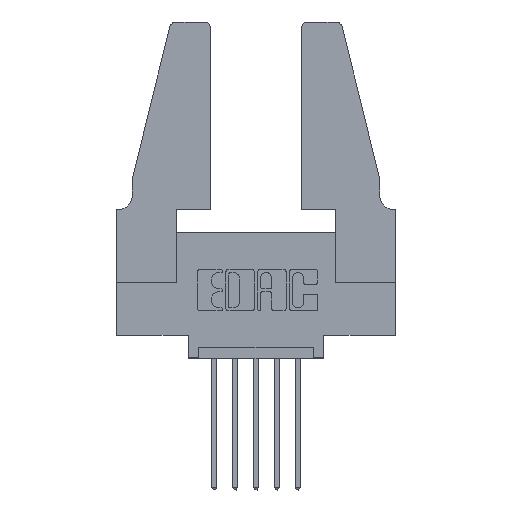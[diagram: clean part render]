
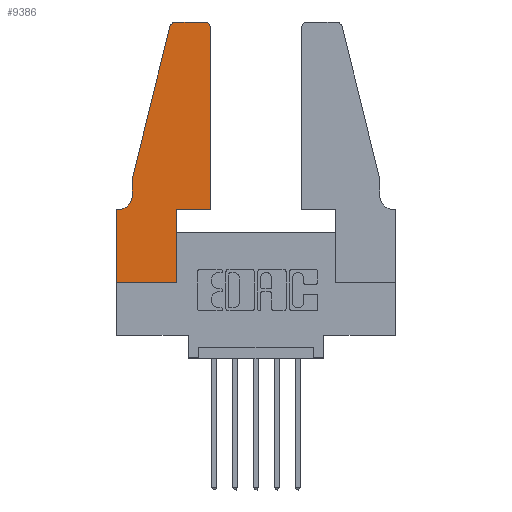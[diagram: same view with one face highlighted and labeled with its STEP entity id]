
A CAD part, top view. The second image highlights one B-rep face of the part: STEP entity #9386.
In plain terms, the highlighted planar face has unit normal (0, 0, 1).
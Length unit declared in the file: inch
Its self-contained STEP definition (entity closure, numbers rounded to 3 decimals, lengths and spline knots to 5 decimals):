
#49 = FACE_OUTER_BOUND ( 'NONE', #9135, .T. ) ;
#96 = EDGE_CURVE ( 'NONE', #5840, #1678, #9204, .T. ) ;
#103 = AXIS2_PLACEMENT_3D ( 'NONE', #2315, #10703, #559 ) ;
#222 = CARTESIAN_POINT ( 'NONE',  ( 0., 0.35, 0.37 ) ) ;
#270 = CARTESIAN_POINT ( 'NONE',  ( 0.4505, 0.35, 0.37 ) ) ;
#273 = VERTEX_POINT ( 'NONE', #8104 ) ;
#385 = AXIS2_PLACEMENT_3D ( 'NONE', #4995, #5031, #11006 ) ;
#559 = DIRECTION ( 'NONE',  ( 1., 0., 0. ) ) ;
#604 = DIRECTION ( 'NONE',  ( 0., -1., 0. ) ) ;
#610 = AXIS2_PLACEMENT_3D ( 'NONE', #1823, #6894, #1903 ) ;
#1371 = CARTESIAN_POINT ( 'NONE',  ( 0.0755, 0.5, 0.37 ) ) ;
#1377 = LINE ( 'NONE', #1539, #10598 ) ;
#1414 = EDGE_CURVE ( 'NONE', #4441, #5283, #2068, .T. ) ;
#1539 = CARTESIAN_POINT ( 'NONE',  ( 0.4505, 0.35, 0.37 ) ) ;
#1623 = VERTEX_POINT ( 'NONE', #5272 ) ;
#1678 = VERTEX_POINT ( 'NONE', #5343 ) ;
#1774 = CARTESIAN_POINT ( 'NONE',  ( 0.25487, 1.22718, 0.37 ) ) ;
#1823 = CARTESIAN_POINT ( 'NONE',  ( 0.284, 1.22, 0.37 ) ) ;
#1831 = VECTOR ( 'NONE', #3456, 39.37008 ) ;
#1847 = PLANE ( 'NONE',  #2096 ) ;
#1903 = DIRECTION ( 'NONE',  ( 1., 0., 0. ) ) ;
#1914 = ORIENTED_EDGE ( 'NONE', *, *, #96, .T. ) ;
#2068 = LINE ( 'NONE', #2336, #10095 ) ;
#2096 = AXIS2_PLACEMENT_3D ( 'NONE', #222, #3587, #8772 ) ;
#2315 = CARTESIAN_POINT ( 'NONE',  ( 0.4205, 1.22, 0.37 ) ) ;
#2336 = CARTESIAN_POINT ( 'NONE',  ( 0.2865, 0.35, 0.37 ) ) ;
#2390 = EDGE_CURVE ( 'NONE', #5383, #3233, #2455, .T. ) ;
#2402 = DIRECTION ( 'NONE',  ( 0., 1., 0. ) ) ;
#2405 = DIRECTION ( 'NONE',  ( 0., 1., 0. ) ) ;
#2445 = ORIENTED_EDGE ( 'NONE', *, *, #2390, .T. ) ;
#2455 = CIRCLE ( 'NONE', #103, 0.03 ) ;
#2589 = CARTESIAN_POINT ( 'NONE',  ( 0.4505, 0.35, 0.37 ) ) ;
#2709 = ORIENTED_EDGE ( 'NONE', *, *, #10622, .T. ) ;
#2716 = VECTOR ( 'NONE', #604, 39.37008 ) ;
#2781 = ORIENTED_EDGE ( 'NONE', *, *, #1414, .T. ) ;
#3050 = EDGE_CURVE ( 'NONE', #10667, #5383, #1377, .T. ) ;
#3233 = VERTEX_POINT ( 'NONE', #9500 ) ;
#3453 = EDGE_CURVE ( 'NONE', #1678, #8288, #4985, .T. ) ;
#3456 = DIRECTION ( 'NONE',  ( 1., 0., 0. ) ) ;
#3461 = EDGE_CURVE ( 'NONE', #8288, #7894, #7801, .T. ) ;
#3587 = DIRECTION ( 'NONE',  ( 0., 0., 1. ) ) ;
#4040 = VECTOR ( 'NONE', #5725, 39.37008 ) ;
#4083 = DIRECTION ( 'NONE',  ( 0., -1., 0. ) ) ;
#4408 = ORIENTED_EDGE ( 'NONE', *, *, #9674, .T. ) ;
#4441 = VERTEX_POINT ( 'NONE', #5836 ) ;
#4565 = CARTESIAN_POINT ( 'NONE',  ( 0.0755, 0.35, 0.37 ) ) ;
#4654 = ORIENTED_EDGE ( 'NONE', *, *, #4861, .T. ) ;
#4839 = LINE ( 'NONE', #10012, #5105 ) ;
#4861 = EDGE_CURVE ( 'NONE', #3233, #273, #6295, .T. ) ;
#4869 = CARTESIAN_POINT ( 'NONE',  ( 0.2605, 1.25, 0.37 ) ) ;
#4985 = LINE ( 'NONE', #1371, #2716 ) ;
#4995 = CARTESIAN_POINT ( 'NONE',  ( 0.0055, 0.42, 0.37 ) ) ;
#5031 = DIRECTION ( 'NONE',  ( 0., 0., -1. ) ) ;
#5105 = VECTOR ( 'NONE', #4083, 39.37008 ) ;
#5272 = CARTESIAN_POINT ( 'NONE',  ( 0., 0., 0.37 ) ) ;
#5283 = VERTEX_POINT ( 'NONE', #6942 ) ;
#5343 = CARTESIAN_POINT ( 'NONE',  ( 0.0755, 0.5, 0.37 ) ) ;
#5383 = VERTEX_POINT ( 'NONE', #10926 ) ;
#5588 = LINE ( 'NONE', #2589, #1831 ) ;
#5725 = DIRECTION ( 'NONE',  ( -1., 0., 0. ) ) ;
#5743 = CARTESIAN_POINT ( 'NONE',  ( 0.0055, 0.35, 0.37 ) ) ;
#5749 = ORIENTED_EDGE ( 'NONE', *, *, #9790, .T. ) ;
#5775 = LINE ( 'NONE', #9478, #6170 ) ;
#5809 = CIRCLE ( 'NONE', #610, 0.03 ) ;
#5836 = CARTESIAN_POINT ( 'NONE',  ( 0.2865, 0., 0.37 ) ) ;
#5840 = VERTEX_POINT ( 'NONE', #1774 ) ;
#5991 = VECTOR ( 'NONE', #9043, 39.37008 ) ;
#5999 = DIRECTION ( 'NONE',  ( 1., 0., 0. ) ) ;
#6087 = EDGE_CURVE ( 'NONE', #5283, #10667, #5588, .T. ) ;
#6170 = VECTOR ( 'NONE', #5999, 39.37008 ) ;
#6295 = LINE ( 'NONE', #4869, #4040 ) ;
#6690 = CARTESIAN_POINT ( 'NONE',  ( 0., 0.35, 0.37 ) ) ;
#6719 = CARTESIAN_POINT ( 'NONE',  ( 0.0755, 0.42, 0.37 ) ) ;
#6894 = DIRECTION ( 'NONE',  ( 0., 0., 1. ) ) ;
#6942 = CARTESIAN_POINT ( 'NONE',  ( 0.2865, 0.35, 0.37 ) ) ;
#6985 = VERTEX_POINT ( 'NONE', #6690 ) ;
#7042 = ORIENTED_EDGE ( 'NONE', *, *, #8591, .T. ) ;
#7087 = DIRECTION ( 'NONE',  ( -1., 0., 0. ) ) ;
#7113 = ORIENTED_EDGE ( 'NONE', *, *, #6087, .T. ) ;
#7625 = ORIENTED_EDGE ( 'NONE', *, *, #3461, .T. ) ;
#7691 = LINE ( 'NONE', #4565, #10081 ) ;
#7801 = CIRCLE ( 'NONE', #385, 0.07 ) ;
#7894 = VERTEX_POINT ( 'NONE', #5743 ) ;
#8104 = CARTESIAN_POINT ( 'NONE',  ( 0.284, 1.25, 0.37 ) ) ;
#8288 = VERTEX_POINT ( 'NONE', #6719 ) ;
#8591 = EDGE_CURVE ( 'NONE', #273, #5840, #5809, .T. ) ;
#8772 = DIRECTION ( 'NONE',  ( 1., 0., 0. ) ) ;
#8961 = CARTESIAN_POINT ( 'NONE',  ( 0.0755, 0.5, 0.37 ) ) ;
#9043 = DIRECTION ( 'NONE',  ( -0.239, -0.971, 0. ) ) ;
#9135 = EDGE_LOOP ( 'NONE', ( #4654, #7042, #1914, #10980, #7625, #2709, #4408, #5749, #2781, #7113, #9466, #2445 ) ) ;
#9204 = LINE ( 'NONE', #8961, #5991 ) ;
#9386 = ADVANCED_FACE ( 'NONE', ( #49 ), #1847, .T. ) ;
#9466 = ORIENTED_EDGE ( 'NONE', *, *, #3050, .T. ) ;
#9478 = CARTESIAN_POINT ( 'NONE',  ( 0., 0., 0.37 ) ) ;
#9500 = CARTESIAN_POINT ( 'NONE',  ( 0.4205, 1.25, 0.37 ) ) ;
#9674 = EDGE_CURVE ( 'NONE', #6985, #1623, #4839, .T. ) ;
#9790 = EDGE_CURVE ( 'NONE', #1623, #4441, #5775, .T. ) ;
#10012 = CARTESIAN_POINT ( 'NONE',  ( 0., 0., 0.37 ) ) ;
#10081 = VECTOR ( 'NONE', #7087, 39.37008 ) ;
#10095 = VECTOR ( 'NONE', #2402, 39.37008 ) ;
#10598 = VECTOR ( 'NONE', #2405, 39.37008 ) ;
#10622 = EDGE_CURVE ( 'NONE', #7894, #6985, #7691, .T. ) ;
#10667 = VERTEX_POINT ( 'NONE', #270 ) ;
#10703 = DIRECTION ( 'NONE',  ( 0., 0., 1. ) ) ;
#10926 = CARTESIAN_POINT ( 'NONE',  ( 0.4505, 1.22, 0.37 ) ) ;
#10980 = ORIENTED_EDGE ( 'NONE', *, *, #3453, .T. ) ;
#11006 = DIRECTION ( 'NONE',  ( -1., 0., 0. ) ) ;
